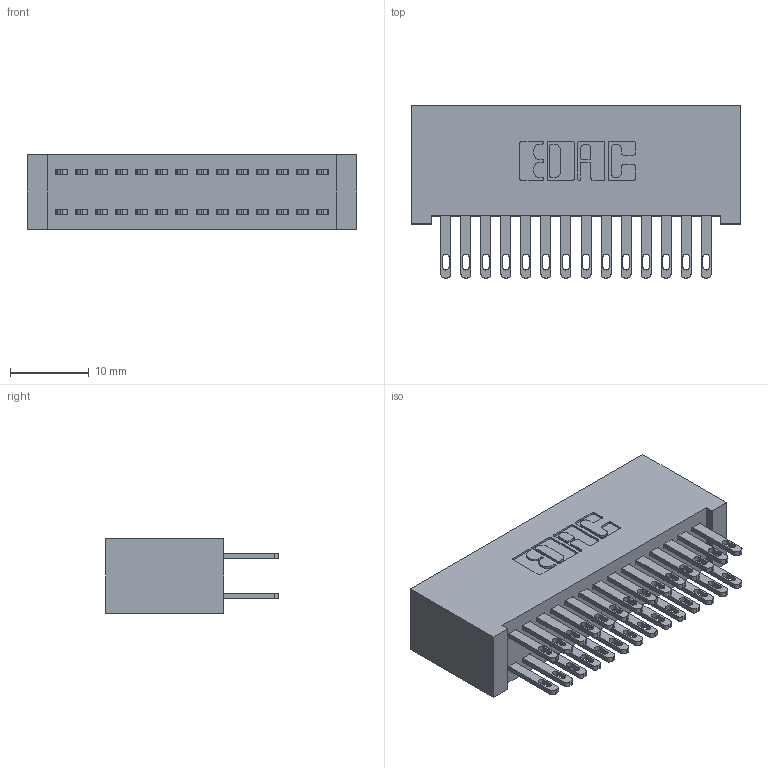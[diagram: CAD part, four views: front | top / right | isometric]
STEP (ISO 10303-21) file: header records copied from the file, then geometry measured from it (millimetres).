
FILE_DESCRIPTION (( 'STEP AP203' ), '1' );
FILE_NAME ('892-028-500-201.STEP', '2020-09-21T14:53:47', ( '' ), ( '' ), 'SwSTEP 2.0', 'SolidWorks 2020', '' );
FILE_SCHEMA (( 'CONFIG_CONTROL_DESIGN' ));
Length unit declared in the file: inch
Products named in the file (3): 345-292-001_345-293-100; 892-028-500-201; 842 Part_Lugless
Assembly tree (29 placements, depth 2):
  892-028-500-201
    842 Part_Lugless
    345-292-001_345-293-100  x28
Bounding box: 41.81 x 21.85 x 9.4 mm (x, y, z)
Volume: 4149 mm3; surface area: 6777.9 mm2
Topology: 29 solids, 29 shells, 1446 faces, 4391 edges, 2926 vertices
Faces by surface type: plane 902, cylinder 544
Entity records: 12149 total; most frequent: CARTESIAN_POINT 2042, ORIENTED_EDGE 1978, DIRECTION 1789, EDGE_CURVE 989, VECTOR 865, LINE 865, VERTEX_POINT 658, AXIS2_PLACEMENT_3D 462
